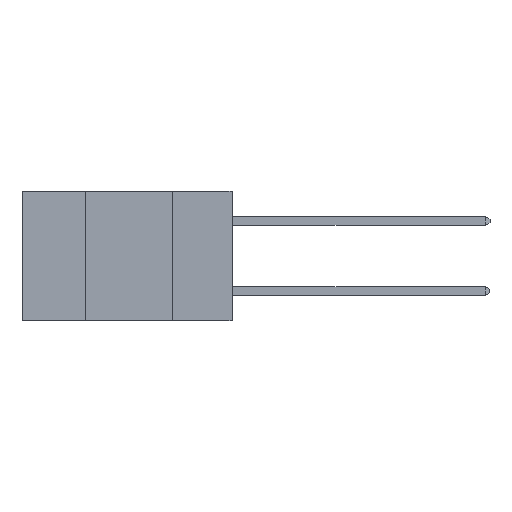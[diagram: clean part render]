
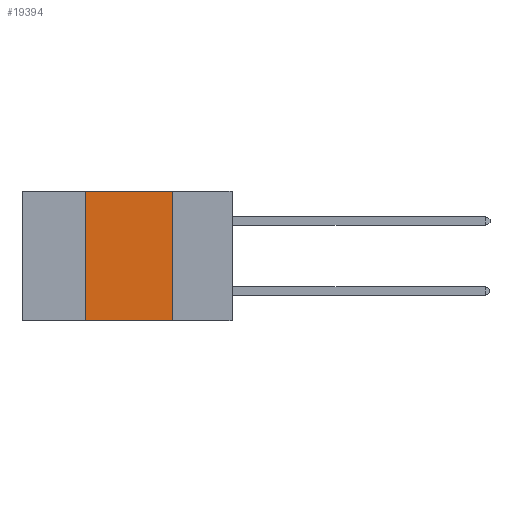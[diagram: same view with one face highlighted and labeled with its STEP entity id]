
A CAD part, left-side view. The second image highlights one B-rep face of the part: STEP entity #19394.
In plain terms, the highlighted planar face has unit normal (-1, 0, 0).
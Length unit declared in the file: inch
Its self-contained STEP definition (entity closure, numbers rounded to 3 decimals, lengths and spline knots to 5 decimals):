
#406 = VECTOR ( 'NONE', #16744, 39.37008 ) ;
#1183 = CARTESIAN_POINT ( 'NONE',  ( 0., 0.6, -0.37 ) ) ;
#1442 = LINE ( 'NONE', #15261, #406 ) ;
#2835 = DIRECTION ( 'NONE',  ( 0., -1., 0. ) ) ;
#3319 = DIRECTION ( 'NONE',  ( 0., -1., 0. ) ) ;
#5758 = CARTESIAN_POINT ( 'NONE',  ( 0., 0.42, 0. ) ) ;
#6900 = PLANE ( 'NONE',  #19335 ) ;
#6943 = CARTESIAN_POINT ( 'NONE',  ( 0., 0.17, -0.37 ) ) ;
#7253 = EDGE_CURVE ( 'NONE', #9283, #8021, #8304, .T. ) ;
#8021 = VERTEX_POINT ( 'NONE', #5758 ) ;
#8098 = EDGE_CURVE ( 'NONE', #13579, #11307, #1442, .T. ) ;
#8304 = LINE ( 'NONE', #8529, #16108 ) ;
#8447 = DIRECTION ( 'NONE',  ( 1., 0., 0. ) ) ;
#8529 = CARTESIAN_POINT ( 'NONE',  ( 0., 0.42, 0. ) ) ;
#8736 = LINE ( 'NONE', #1183, #16518 ) ;
#8753 = EDGE_CURVE ( 'NONE', #9283, #11307, #8736, .T. ) ;
#9161 = FACE_OUTER_BOUND ( 'NONE', #10995, .T. ) ;
#9283 = VERTEX_POINT ( 'NONE', #10605 ) ;
#10605 = CARTESIAN_POINT ( 'NONE',  ( 0., 0.42, -0.37 ) ) ;
#10995 = EDGE_LOOP ( 'NONE', ( #17461, #15583, #15000, #16746 ) ) ;
#11307 = VERTEX_POINT ( 'NONE', #6943 ) ;
#12218 = CARTESIAN_POINT ( 'NONE',  ( 0., 0.17, 0. ) ) ;
#13579 = VERTEX_POINT ( 'NONE', #12218 ) ;
#14127 = CARTESIAN_POINT ( 'NONE',  ( 0., 0.6, 0. ) ) ;
#15000 = ORIENTED_EDGE ( 'NONE', *, *, #7253, .F. ) ;
#15261 = CARTESIAN_POINT ( 'NONE',  ( 0., 0.17, 0. ) ) ;
#15583 = ORIENTED_EDGE ( 'NONE', *, *, #16132, .F. ) ;
#16108 = VECTOR ( 'NONE', #17713, 39.37008 ) ;
#16132 = EDGE_CURVE ( 'NONE', #8021, #13579, #17916, .T. ) ;
#16518 = VECTOR ( 'NONE', #2835, 39.37008 ) ;
#16744 = DIRECTION ( 'NONE',  ( 0., 0., -1. ) ) ;
#16746 = ORIENTED_EDGE ( 'NONE', *, *, #8753, .T. ) ;
#17027 = VECTOR ( 'NONE', #3319, 39.37008 ) ;
#17461 = ORIENTED_EDGE ( 'NONE', *, *, #8098, .F. ) ;
#17635 = CARTESIAN_POINT ( 'NONE',  ( 0., 0.6, 0. ) ) ;
#17713 = DIRECTION ( 'NONE',  ( 0., 0., 1. ) ) ;
#17916 = LINE ( 'NONE', #14127, #17027 ) ;
#19088 = DIRECTION ( 'NONE',  ( 0., 0., -1. ) ) ;
#19335 = AXIS2_PLACEMENT_3D ( 'NONE', #17635, #8447, #19088 ) ;
#19394 = ADVANCED_FACE ( 'NONE', ( #9161 ), #6900, .F. ) ;
